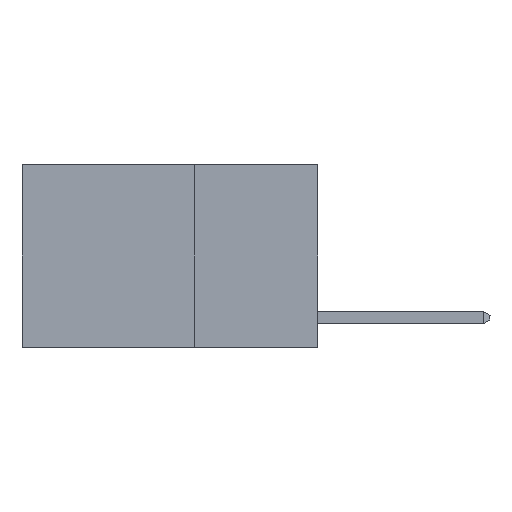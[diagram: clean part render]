
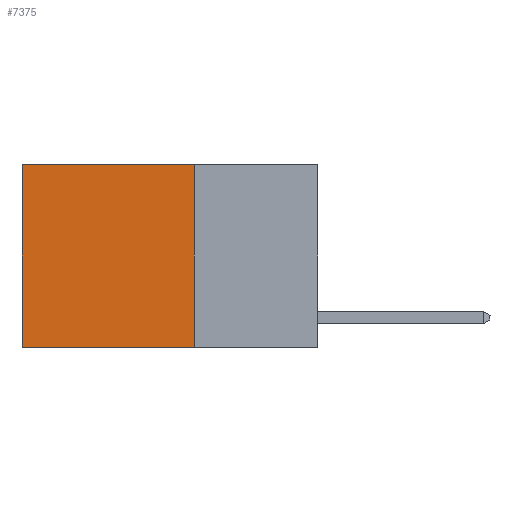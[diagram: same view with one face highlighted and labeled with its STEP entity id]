
A CAD part, left-side view. The second image highlights one B-rep face of the part: STEP entity #7375.
In plain terms, the highlighted planar face has unit normal (-1, 0, 0).
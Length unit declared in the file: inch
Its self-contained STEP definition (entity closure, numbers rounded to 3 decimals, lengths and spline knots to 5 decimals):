
#82 = CARTESIAN_POINT ( 'NONE',  ( 0.2625, 0.25, 0. ) ) ;
#232 = DIRECTION ( 'NONE',  ( 0., 0., -1. ) ) ;
#1238 = AXIS2_PLACEMENT_3D ( 'NONE', #12053, #27921, #16968 ) ;
#1755 = LINE ( 'NONE', #10993, #27944 ) ;
#2197 = CARTESIAN_POINT ( 'NONE',  ( 0.2625, 0.25, -0.37 ) ) ;
#2648 = CARTESIAN_POINT ( 'NONE',  ( 0.2625, 0.6, 0. ) ) ;
#2764 = EDGE_CURVE ( 'NONE', #13118, #14753, #9673, .T. ) ;
#3562 = ORIENTED_EDGE ( 'NONE', *, *, #2764, .T. ) ;
#4561 = EDGE_CURVE ( 'NONE', #6024, #13118, #1755, .T. ) ;
#4605 = ORIENTED_EDGE ( 'NONE', *, *, #5967, .F. ) ;
#5448 = ORIENTED_EDGE ( 'NONE', *, *, #8409, .F. ) ;
#5516 = VECTOR ( 'NONE', #232, 39.37008 ) ;
#5967 = EDGE_CURVE ( 'NONE', #22096, #14753, #26320, .T. ) ;
#6024 = VERTEX_POINT ( 'NONE', #15499 ) ;
#7375 = ADVANCED_FACE ( 'NONE', ( #27634 ), #9887, .F. ) ;
#8409 = EDGE_CURVE ( 'NONE', #6024, #22096, #19744, .T. ) ;
#9393 = EDGE_LOOP ( 'NONE', ( #3562, #4605, #5448, #19771 ) ) ;
#9673 = LINE ( 'NONE', #9965, #19130 ) ;
#9887 = PLANE ( 'NONE',  #1238 ) ;
#9965 = CARTESIAN_POINT ( 'NONE',  ( 0.2625, 0.6, 0. ) ) ;
#10993 = CARTESIAN_POINT ( 'NONE',  ( 0.2625, 0.25, 0. ) ) ;
#12053 = CARTESIAN_POINT ( 'NONE',  ( 0.2625, 0.25, 0. ) ) ;
#13118 = VERTEX_POINT ( 'NONE', #2648 ) ;
#14753 = VERTEX_POINT ( 'NONE', #27165 ) ;
#14925 = DIRECTION ( 'NONE',  ( 0., 1., 0. ) ) ;
#15499 = CARTESIAN_POINT ( 'NONE',  ( 0.2625, 0.25, 0. ) ) ;
#16098 = CARTESIAN_POINT ( 'NONE',  ( 0.2625, 0.25, -0.37 ) ) ;
#16968 = DIRECTION ( 'NONE',  ( 0., 0., -1. ) ) ;
#18940 = DIRECTION ( 'NONE',  ( 0., 0., -1. ) ) ;
#19130 = VECTOR ( 'NONE', #18940, 39.37008 ) ;
#19744 = LINE ( 'NONE', #82, #5516 ) ;
#19771 = ORIENTED_EDGE ( 'NONE', *, *, #4561, .T. ) ;
#22096 = VERTEX_POINT ( 'NONE', #16098 ) ;
#26320 = LINE ( 'NONE', #2197, #28011 ) ;
#27165 = CARTESIAN_POINT ( 'NONE',  ( 0.2625, 0.6, -0.37 ) ) ;
#27634 = FACE_OUTER_BOUND ( 'NONE', #9393, .T. ) ;
#27921 = DIRECTION ( 'NONE',  ( 1., 0., 0. ) ) ;
#27944 = VECTOR ( 'NONE', #14925, 39.37008 ) ;
#28011 = VECTOR ( 'NONE', #28336, 39.37008 ) ;
#28336 = DIRECTION ( 'NONE',  ( 0., 1., 0. ) ) ;
